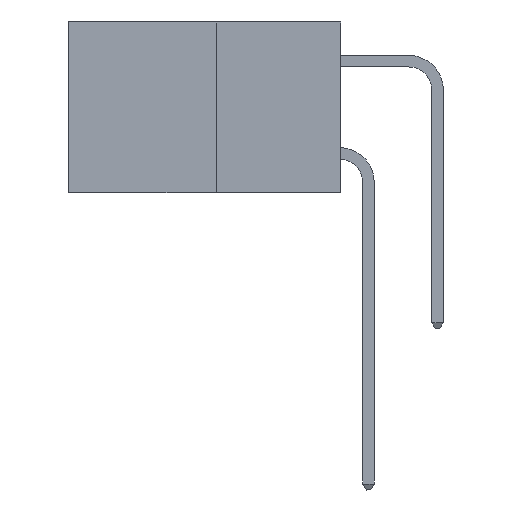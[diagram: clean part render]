
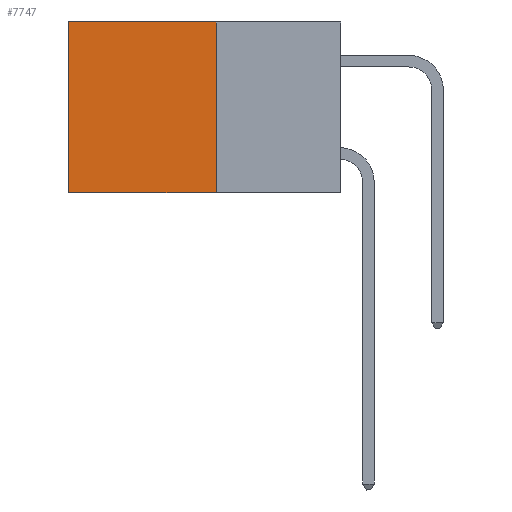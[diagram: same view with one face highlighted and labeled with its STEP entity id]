
A CAD part, left-side view. The second image highlights one B-rep face of the part: STEP entity #7747.
In plain terms, the highlighted planar face has unit normal (-1, 0, 0).
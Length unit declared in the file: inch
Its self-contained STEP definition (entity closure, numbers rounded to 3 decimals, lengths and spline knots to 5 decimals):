
#57 = CARTESIAN_POINT ( 'NONE',  ( 0.277, 0.27, -0.37 ) ) ;
#244 = CARTESIAN_POINT ( 'NONE',  ( 0.277, 0.27, -0.37 ) ) ;
#3309 = CARTESIAN_POINT ( 'NONE',  ( 0.277, 0.59, -0.37 ) ) ;
#3999 = VECTOR ( 'NONE', #18753, 39.37008 ) ;
#4499 = DIRECTION ( 'NONE',  ( 0., 0., -1. ) ) ;
#4798 = DIRECTION ( 'NONE',  ( 0., 0., -1. ) ) ;
#5119 = ORIENTED_EDGE ( 'NONE', *, *, #6821, .T. ) ;
#6274 = VERTEX_POINT ( 'NONE', #18191 ) ;
#6821 = EDGE_CURVE ( 'NONE', #12316, #11715, #15347, .T. ) ;
#7408 = VECTOR ( 'NONE', #12025, 39.37008 ) ;
#7747 = ADVANCED_FACE ( 'NONE', ( #14834 ), #10389, .F. ) ;
#7848 = ORIENTED_EDGE ( 'NONE', *, *, #12965, .T. ) ;
#7880 = CARTESIAN_POINT ( 'NONE',  ( 0.277, 0.59, 0. ) ) ;
#7982 = LINE ( 'NONE', #57, #3999 ) ;
#9164 = CARTESIAN_POINT ( 'NONE',  ( 0.277, 0.27, 0. ) ) ;
#10085 = DIRECTION ( 'NONE',  ( 0., 0., -1. ) ) ;
#10102 = DIRECTION ( 'NONE',  ( 1., 0., 0. ) ) ;
#10199 = EDGE_CURVE ( 'NONE', #11629, #6274, #7982, .T. ) ;
#10389 = PLANE ( 'NONE',  #16356 ) ;
#10431 = CARTESIAN_POINT ( 'NONE',  ( 0.277, 0.27, -0.37 ) ) ;
#10879 = VECTOR ( 'NONE', #4499, 39.37008 ) ;
#11629 = VERTEX_POINT ( 'NONE', #244 ) ;
#11715 = VERTEX_POINT ( 'NONE', #7880 ) ;
#11920 = LINE ( 'NONE', #3309, #15936 ) ;
#12025 = DIRECTION ( 'NONE',  ( 0., 1., 0. ) ) ;
#12316 = VERTEX_POINT ( 'NONE', #9164 ) ;
#12965 = EDGE_CURVE ( 'NONE', #11715, #6274, #11920, .T. ) ;
#13032 = ORIENTED_EDGE ( 'NONE', *, *, #10199, .F. ) ;
#14834 = FACE_OUTER_BOUND ( 'NONE', #16108, .T. ) ;
#15322 = LINE ( 'NONE', #18009, #10879 ) ;
#15347 = LINE ( 'NONE', #15759, #7408 ) ;
#15675 = ORIENTED_EDGE ( 'NONE', *, *, #16455, .F. ) ;
#15759 = CARTESIAN_POINT ( 'NONE',  ( 0.277, 0.27, 0. ) ) ;
#15936 = VECTOR ( 'NONE', #4798, 39.37008 ) ;
#16108 = EDGE_LOOP ( 'NONE', ( #7848, #13032, #15675, #5119 ) ) ;
#16356 = AXIS2_PLACEMENT_3D ( 'NONE', #10431, #10102, #10085 ) ;
#16455 = EDGE_CURVE ( 'NONE', #12316, #11629, #15322, .T. ) ;
#18009 = CARTESIAN_POINT ( 'NONE',  ( 0.277, 0.27, -0.37 ) ) ;
#18191 = CARTESIAN_POINT ( 'NONE',  ( 0.277, 0.59, -0.37 ) ) ;
#18753 = DIRECTION ( 'NONE',  ( 0., 1., 0. ) ) ;
